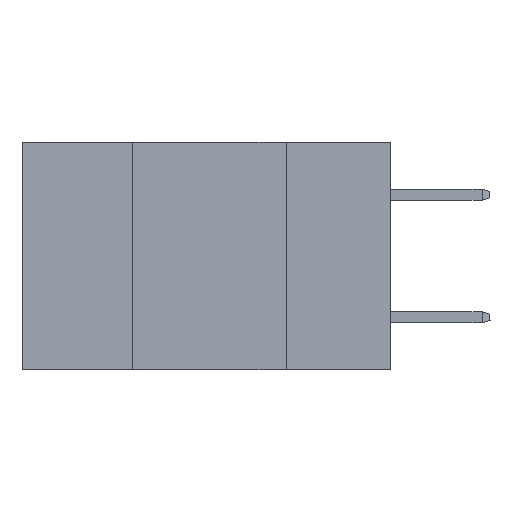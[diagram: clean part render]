
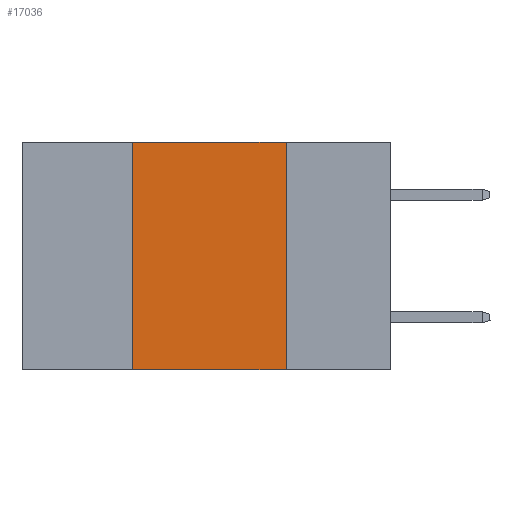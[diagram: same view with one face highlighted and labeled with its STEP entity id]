
A CAD part, left-side view. The second image highlights one B-rep face of the part: STEP entity #17036.
In plain terms, the highlighted planar face has unit normal (-1, 0, 0).
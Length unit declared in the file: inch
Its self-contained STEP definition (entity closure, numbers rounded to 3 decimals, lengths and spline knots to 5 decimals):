
#582 = DIRECTION ( 'NONE',  ( 0., 0., -1. ) ) ;
#979 = EDGE_CURVE ( 'NONE', #1351, #5946, #13220, .T. ) ;
#1115 = EDGE_LOOP ( 'NONE', ( #2415, #3672, #22699, #8176 ) ) ;
#1351 = VERTEX_POINT ( 'NONE', #15538 ) ;
#2246 = LINE ( 'NONE', #7000, #19591 ) ;
#2415 = ORIENTED_EDGE ( 'NONE', *, *, #15432, .F. ) ;
#3672 = ORIENTED_EDGE ( 'NONE', *, *, #21035, .F. ) ;
#3910 = CARTESIAN_POINT ( 'NONE',  ( 0., 0.6, -0.37 ) ) ;
#3937 = CARTESIAN_POINT ( 'NONE',  ( 0., 0.6, 0. ) ) ;
#5946 = VERTEX_POINT ( 'NONE', #17790 ) ;
#6057 = DIRECTION ( 'NONE',  ( 0., 0., 1. ) ) ;
#6892 = CARTESIAN_POINT ( 'NONE',  ( 0., 0.42, 0. ) ) ;
#7000 = CARTESIAN_POINT ( 'NONE',  ( 0., 0.6, 0. ) ) ;
#8130 = DIRECTION ( 'NONE',  ( 0., -1., 0. ) ) ;
#8176 = ORIENTED_EDGE ( 'NONE', *, *, #10364, .T. ) ;
#10364 = EDGE_CURVE ( 'NONE', #1351, #12314, #24104, .T. ) ;
#12314 = VERTEX_POINT ( 'NONE', #16309 ) ;
#12611 = DIRECTION ( 'NONE',  ( 1., 0., 0. ) ) ;
#13010 = LINE ( 'NONE', #13448, #22470 ) ;
#13220 = LINE ( 'NONE', #6892, #26758 ) ;
#13448 = CARTESIAN_POINT ( 'NONE',  ( 0., 0.17, 0. ) ) ;
#15432 = EDGE_CURVE ( 'NONE', #19017, #12314, #13010, .T. ) ;
#15538 = CARTESIAN_POINT ( 'NONE',  ( 0., 0.42, -0.37 ) ) ;
#16309 = CARTESIAN_POINT ( 'NONE',  ( 0., 0.17, -0.37 ) ) ;
#16439 = AXIS2_PLACEMENT_3D ( 'NONE', #3937, #12611, #27762 ) ;
#17036 = ADVANCED_FACE ( 'NONE', ( #21524 ), #19036, .F. ) ;
#17414 = CARTESIAN_POINT ( 'NONE',  ( 0., 0.17, 0. ) ) ;
#17790 = CARTESIAN_POINT ( 'NONE',  ( 0., 0.42, 0. ) ) ;
#19017 = VERTEX_POINT ( 'NONE', #17414 ) ;
#19036 = PLANE ( 'NONE',  #16439 ) ;
#19591 = VECTOR ( 'NONE', #24299, 39.37008 ) ;
#21035 = EDGE_CURVE ( 'NONE', #5946, #19017, #2246, .T. ) ;
#21382 = VECTOR ( 'NONE', #8130, 39.37008 ) ;
#21524 = FACE_OUTER_BOUND ( 'NONE', #1115, .T. ) ;
#22470 = VECTOR ( 'NONE', #582, 39.37008 ) ;
#22699 = ORIENTED_EDGE ( 'NONE', *, *, #979, .F. ) ;
#24104 = LINE ( 'NONE', #3910, #21382 ) ;
#24299 = DIRECTION ( 'NONE',  ( 0., -1., 0. ) ) ;
#26758 = VECTOR ( 'NONE', #6057, 39.37008 ) ;
#27762 = DIRECTION ( 'NONE',  ( 0., 0., -1. ) ) ;
